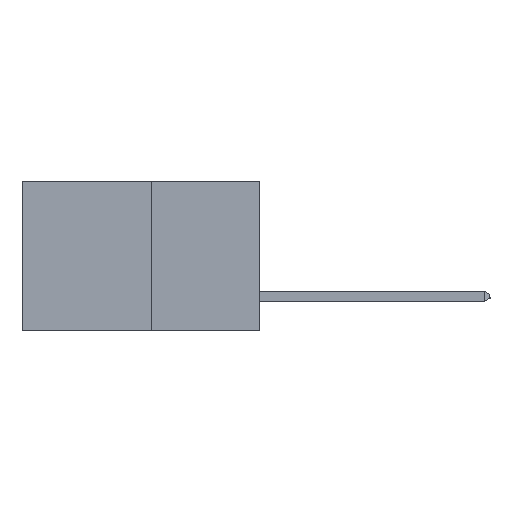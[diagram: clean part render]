
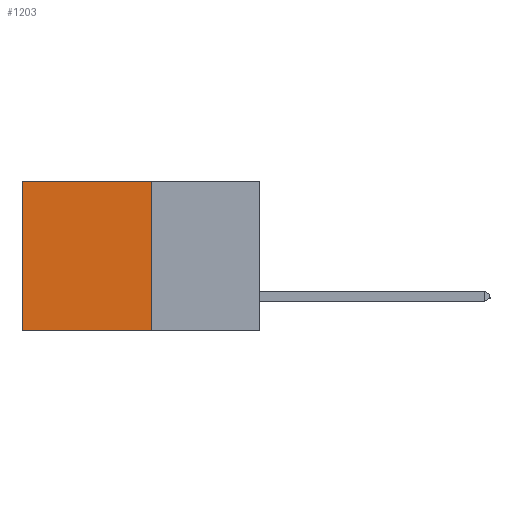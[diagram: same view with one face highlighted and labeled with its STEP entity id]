
A CAD part, left-side view. The second image highlights one B-rep face of the part: STEP entity #1203.
In plain terms, the highlighted planar face has unit normal (-1, 0, 0).
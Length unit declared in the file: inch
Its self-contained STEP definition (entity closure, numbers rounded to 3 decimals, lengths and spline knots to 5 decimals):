
#291 = DIRECTION ( 'NONE',  ( 0., 0., -1. ) ) ;
#544 = EDGE_CURVE ( 'NONE', #5214, #9343, #11452, .T. ) ;
#1203 = ADVANCED_FACE ( 'NONE', ( #11162 ), #7652, .F. ) ;
#1296 = EDGE_LOOP ( 'NONE', ( #1361, #6641, #9010, #1662 ) ) ;
#1330 = EDGE_CURVE ( 'NONE', #10573, #9343, #11292, .T. ) ;
#1361 = ORIENTED_EDGE ( 'NONE', *, *, #1330, .T. ) ;
#1389 = CARTESIAN_POINT ( 'NONE',  ( 0.277, 0.27, -0.37 ) ) ;
#1662 = ORIENTED_EDGE ( 'NONE', *, *, #6400, .T. ) ;
#1897 = VECTOR ( 'NONE', #9527, 39.37008 ) ;
#2376 = EDGE_CURVE ( 'NONE', #10801, #5214, #5905, .T. ) ;
#2400 = VECTOR ( 'NONE', #3638, 39.37008 ) ;
#2625 = VECTOR ( 'NONE', #5234, 39.37008 ) ;
#3638 = DIRECTION ( 'NONE',  ( 0., 1., 0. ) ) ;
#4106 = CARTESIAN_POINT ( 'NONE',  ( 0.277, 0.59, -0.37 ) ) ;
#5214 = VERTEX_POINT ( 'NONE', #12036 ) ;
#5234 = DIRECTION ( 'NONE',  ( 0., 0., -1. ) ) ;
#5905 = LINE ( 'NONE', #1389, #2625 ) ;
#6400 = EDGE_CURVE ( 'NONE', #10801, #10573, #7561, .T. ) ;
#6641 = ORIENTED_EDGE ( 'NONE', *, *, #544, .F. ) ;
#7550 = DIRECTION ( 'NONE',  ( 1., 0., 0. ) ) ;
#7561 = LINE ( 'NONE', #9201, #2400 ) ;
#7652 = PLANE ( 'NONE',  #11561 ) ;
#8840 = CARTESIAN_POINT ( 'NONE',  ( 0.277, 0.59, 0. ) ) ;
#9010 = ORIENTED_EDGE ( 'NONE', *, *, #2376, .F. ) ;
#9060 = VECTOR ( 'NONE', #10283, 39.37008 ) ;
#9201 = CARTESIAN_POINT ( 'NONE',  ( 0.277, 0.27, 0. ) ) ;
#9343 = VERTEX_POINT ( 'NONE', #4106 ) ;
#9527 = DIRECTION ( 'NONE',  ( 0., 1., 0. ) ) ;
#9866 = CARTESIAN_POINT ( 'NONE',  ( 0.277, 0.27, 0. ) ) ;
#10270 = CARTESIAN_POINT ( 'NONE',  ( 0.277, 0.59, -0.37 ) ) ;
#10283 = DIRECTION ( 'NONE',  ( 0., 0., -1. ) ) ;
#10573 = VERTEX_POINT ( 'NONE', #8840 ) ;
#10801 = VERTEX_POINT ( 'NONE', #9866 ) ;
#11162 = FACE_OUTER_BOUND ( 'NONE', #1296, .T. ) ;
#11273 = CARTESIAN_POINT ( 'NONE',  ( 0.277, 0.27, -0.37 ) ) ;
#11292 = LINE ( 'NONE', #10270, #9060 ) ;
#11452 = LINE ( 'NONE', #11968, #1897 ) ;
#11561 = AXIS2_PLACEMENT_3D ( 'NONE', #11273, #7550, #291 ) ;
#11968 = CARTESIAN_POINT ( 'NONE',  ( 0.277, 0.27, -0.37 ) ) ;
#12036 = CARTESIAN_POINT ( 'NONE',  ( 0.277, 0.27, -0.37 ) ) ;
